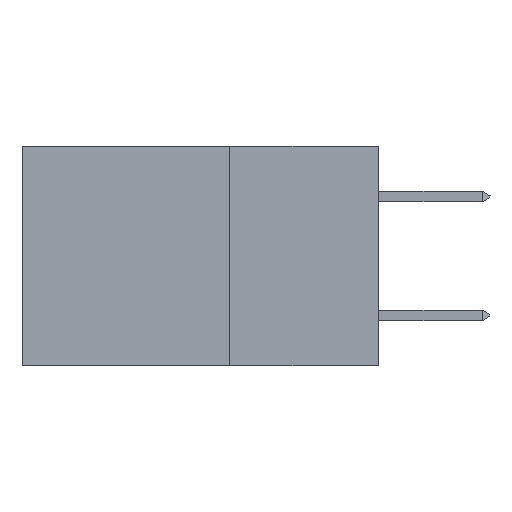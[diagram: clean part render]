
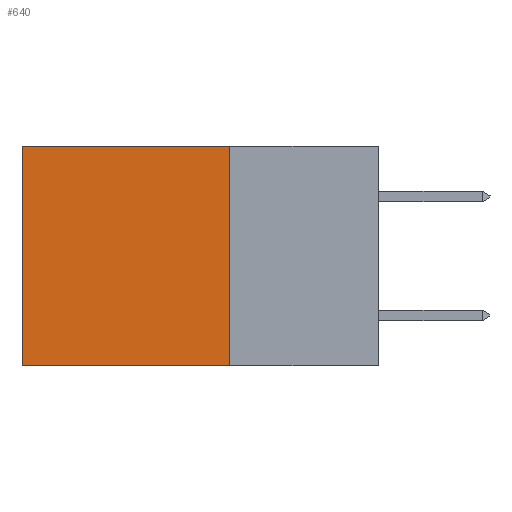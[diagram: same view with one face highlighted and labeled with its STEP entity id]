
A CAD part, left-side view. The second image highlights one B-rep face of the part: STEP entity #640.
In plain terms, the highlighted planar face has unit normal (-1, 0, 0).
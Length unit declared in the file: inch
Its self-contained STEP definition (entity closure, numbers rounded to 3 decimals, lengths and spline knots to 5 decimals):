
#97 = DIRECTION ( 'NONE',  ( 0., 0., -1. ) ) ;
#256 = DIRECTION ( 'NONE',  ( 0., 1., 0. ) ) ;
#640 = ADVANCED_FACE ( 'NONE', ( #8502 ), #9205, .F. ) ;
#817 = EDGE_CURVE ( 'NONE', #8357, #3540, #9331, .T. ) ;
#1076 = EDGE_CURVE ( 'NONE', #7758, #8357, #5249, .T. ) ;
#1124 = ORIENTED_EDGE ( 'NONE', *, *, #8484, .F. ) ;
#1213 = CARTESIAN_POINT ( 'NONE',  ( 0.2615, 0.25, 0. ) ) ;
#1274 = VECTOR ( 'NONE', #3075, 39.37008 ) ;
#1444 = ORIENTED_EDGE ( 'NONE', *, *, #1076, .T. ) ;
#1633 = CARTESIAN_POINT ( 'NONE',  ( 0.2615, 0.25, -0.37 ) ) ;
#1984 = DIRECTION ( 'NONE',  ( 0., 1., 0. ) ) ;
#2329 = LINE ( 'NONE', #8744, #1274 ) ;
#2798 = CARTESIAN_POINT ( 'NONE',  ( 0.2615, 0.6, -0.37 ) ) ;
#3075 = DIRECTION ( 'NONE',  ( 0., 0., -1. ) ) ;
#3153 = VERTEX_POINT ( 'NONE', #10668 ) ;
#3409 = CARTESIAN_POINT ( 'NONE',  ( 0.2615, 0.25, 0. ) ) ;
#3540 = VERTEX_POINT ( 'NONE', #4319 ) ;
#4319 = CARTESIAN_POINT ( 'NONE',  ( 0.2615, 0.6, -0.37 ) ) ;
#4369 = ORIENTED_EDGE ( 'NONE', *, *, #6958, .F. ) ;
#4606 = VECTOR ( 'NONE', #1984, 39.37008 ) ;
#5003 = DIRECTION ( 'NONE',  ( 1., 0., 0. ) ) ;
#5069 = CARTESIAN_POINT ( 'NONE',  ( 0.2615, 0.25, -0.37 ) ) ;
#5249 = LINE ( 'NONE', #1213, #4606 ) ;
#5368 = CARTESIAN_POINT ( 'NONE',  ( 0.2615, 0.6, 0. ) ) ;
#5791 = DIRECTION ( 'NONE',  ( 0., 0., -1. ) ) ;
#6254 = VECTOR ( 'NONE', #256, 39.37008 ) ;
#6796 = AXIS2_PLACEMENT_3D ( 'NONE', #1633, #5003, #5791 ) ;
#6958 = EDGE_CURVE ( 'NONE', #3153, #3540, #9965, .T. ) ;
#7486 = VECTOR ( 'NONE', #97, 39.37008 ) ;
#7758 = VERTEX_POINT ( 'NONE', #3409 ) ;
#7760 = EDGE_LOOP ( 'NONE', ( #9794, #4369, #1124, #1444 ) ) ;
#8357 = VERTEX_POINT ( 'NONE', #5368 ) ;
#8484 = EDGE_CURVE ( 'NONE', #7758, #3153, #2329, .T. ) ;
#8502 = FACE_OUTER_BOUND ( 'NONE', #7760, .T. ) ;
#8744 = CARTESIAN_POINT ( 'NONE',  ( 0.2615, 0.25, -0.37 ) ) ;
#9205 = PLANE ( 'NONE',  #6796 ) ;
#9331 = LINE ( 'NONE', #2798, #7486 ) ;
#9794 = ORIENTED_EDGE ( 'NONE', *, *, #817, .T. ) ;
#9965 = LINE ( 'NONE', #5069, #6254 ) ;
#10668 = CARTESIAN_POINT ( 'NONE',  ( 0.2615, 0.25, -0.37 ) ) ;
